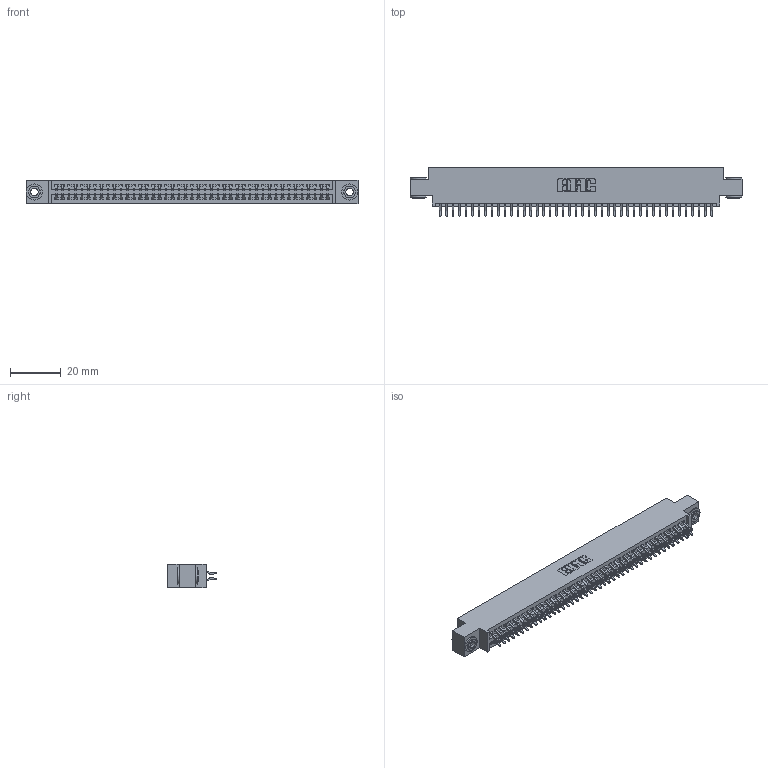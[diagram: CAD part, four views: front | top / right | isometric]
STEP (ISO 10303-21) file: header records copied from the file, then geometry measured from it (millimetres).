
FILE_DESCRIPTION (( 'STEP AP203' ), '1' );
FILE_NAME ('395-086-556-803.STEP', '2018-11-28T22:05:17', ( '' ), ( '' ), 'SwSTEP 2.0', 'SolidWorks 2016', '' );
FILE_SCHEMA (( 'CONFIG_CONTROL_DESIGN' ));
Length unit declared in the file: inch
Products named in the file (4): 345-292-001_556 Tail; 345 Part_0.170 Offset - 0.156 Dia-TH; 345-250-002_345-250-002-102; 395-086-556-803
Assembly tree (89 placements, depth 2):
  395-086-556-803
    345 Part_0.170 Offset - 0.156 Dia-TH
    345-292-001_556 Tail  x86
    345-250-002_345-250-002-102  x2
Bounding box: 130.43 x 19.24 x 9.4 mm (x, y, z)
Volume: 12581.9 mm3; surface area: 18890.6 mm2
Topology: 89 solids, 89 shells, 4984 faces, 14791 edges, 9742 vertices
Faces by surface type: plane 3276, cylinder 1700, cone 8
Entity records: 34606 total; most frequent: CARTESIAN_POINT 5791, ORIENTED_EDGE 5706, DIRECTION 5123, EDGE_CURVE 2853, LINE 2517, VECTOR 2517, VERTEX_POINT 1898, AXIS2_PLACEMENT_3D 1303
